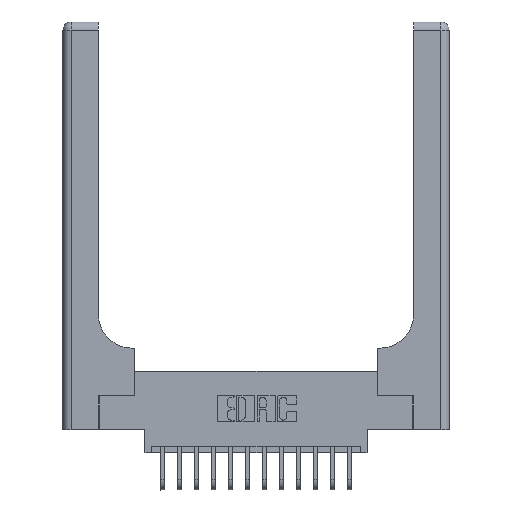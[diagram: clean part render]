
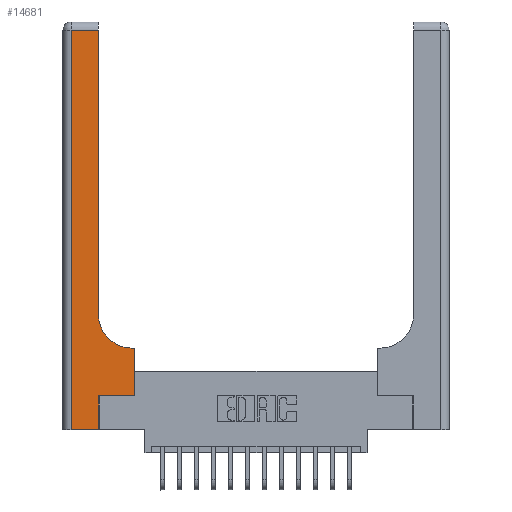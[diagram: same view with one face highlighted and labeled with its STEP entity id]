
A CAD part, top view. The second image highlights one B-rep face of the part: STEP entity #14681.
In plain terms, the highlighted planar face has unit normal (0, 0, 1).
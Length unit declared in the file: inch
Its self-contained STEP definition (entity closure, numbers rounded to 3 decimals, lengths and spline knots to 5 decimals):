
#209 = DIRECTION ( 'NONE',  ( -1., 0., 0. ) ) ;
#928 = CARTESIAN_POINT ( 'NONE',  ( 0., 2.94, 0.37 ) ) ;
#1192 = DIRECTION ( 'NONE',  ( 1., 0., 0. ) ) ;
#1313 = CARTESIAN_POINT ( 'NONE',  ( 0.26, 0.85, 0.37 ) ) ;
#1513 = CARTESIAN_POINT ( 'NONE',  ( 0.26, 3., 0.37 ) ) ;
#1604 = DIRECTION ( 'NONE',  ( 0., -1., 0. ) ) ;
#1934 = LINE ( 'NONE', #13010, #3086 ) ;
#2556 = VECTOR ( 'NONE', #18748, 39.37008 ) ;
#2613 = DIRECTION ( 'NONE',  ( 0., 1., 0. ) ) ;
#2670 = EDGE_CURVE ( 'NONE', #9535, #18361, #16892, .T. ) ;
#2828 = VECTOR ( 'NONE', #11881, 39.37008 ) ;
#3066 = PLANE ( 'NONE',  #6196 ) ;
#3086 = VECTOR ( 'NONE', #2613, 39.37008 ) ;
#3102 = VECTOR ( 'NONE', #6952, 39.37008 ) ;
#3120 = LINE ( 'NONE', #7701, #16442 ) ;
#3555 = ORIENTED_EDGE ( 'NONE', *, *, #8176, .T. ) ;
#3641 = VERTEX_POINT ( 'NONE', #9939 ) ;
#4040 = CARTESIAN_POINT ( 'NONE',  ( 0.528, 0.25, 0.37 ) ) ;
#4149 = CARTESIAN_POINT ( 'NONE',  ( 0.06, 2.94, 0.37 ) ) ;
#4226 = LINE ( 'NONE', #6604, #12489 ) ;
#4505 = ORIENTED_EDGE ( 'NONE', *, *, #17049, .T. ) ;
#4785 = VECTOR ( 'NONE', #12562, 39.37008 ) ;
#5015 = CARTESIAN_POINT ( 'NONE',  ( 0.51, 0.6, 0.37 ) ) ;
#5158 = DIRECTION ( 'NONE',  ( -1., 0., 0. ) ) ;
#5807 = VERTEX_POINT ( 'NONE', #13353 ) ;
#6076 = VERTEX_POINT ( 'NONE', #16192 ) ;
#6196 = AXIS2_PLACEMENT_3D ( 'NONE', #7346, #13395, #209 ) ;
#6457 = VECTOR ( 'NONE', #1192, 39.37008 ) ;
#6515 = ORIENTED_EDGE ( 'NONE', *, *, #12387, .T. ) ;
#6604 = CARTESIAN_POINT ( 'NONE',  ( 0.26, 0.6, 0.37 ) ) ;
#6660 = ORIENTED_EDGE ( 'NONE', *, *, #16191, .T. ) ;
#6952 = DIRECTION ( 'NONE',  ( -1., 0., 0. ) ) ;
#7073 = ORIENTED_EDGE ( 'NONE', *, *, #16228, .T. ) ;
#7172 = ORIENTED_EDGE ( 'NONE', *, *, #15254, .T. ) ;
#7177 = CARTESIAN_POINT ( 'NONE',  ( 0.51, 0.85, 0.37 ) ) ;
#7240 = LINE ( 'NONE', #1513, #2828 ) ;
#7346 = CARTESIAN_POINT ( 'NONE',  ( 0., 3., 0.37 ) ) ;
#7701 = CARTESIAN_POINT ( 'NONE',  ( 0.06, 3., 0.37 ) ) ;
#7970 = VERTEX_POINT ( 'NONE', #8916 ) ;
#8176 = EDGE_CURVE ( 'NONE', #3641, #9535, #4226, .T. ) ;
#8916 = CARTESIAN_POINT ( 'NONE',  ( 0.26, 2.94, 0.37 ) ) ;
#8963 = VERTEX_POINT ( 'NONE', #16200 ) ;
#9535 = VERTEX_POINT ( 'NONE', #5015 ) ;
#9939 = CARTESIAN_POINT ( 'NONE',  ( 0.528, 0.6, 0.37 ) ) ;
#11642 = EDGE_CURVE ( 'NONE', #8963, #5807, #16741, .T. ) ;
#11881 = DIRECTION ( 'NONE',  ( 0., 1., 0. ) ) ;
#12387 = EDGE_CURVE ( 'NONE', #18439, #6076, #16718, .T. ) ;
#12489 = VECTOR ( 'NONE', #5158, 39.37008 ) ;
#12562 = DIRECTION ( 'NONE',  ( 1., 0., 0. ) ) ;
#13010 = CARTESIAN_POINT ( 'NONE',  ( 0.265, 0., 0.37 ) ) ;
#13167 = CARTESIAN_POINT ( 'NONE',  ( 0.06, 0., 0.37 ) ) ;
#13353 = CARTESIAN_POINT ( 'NONE',  ( 0.528, 0.25, 0.37 ) ) ;
#13395 = DIRECTION ( 'NONE',  ( 0., 0., -1. ) ) ;
#13799 = ORIENTED_EDGE ( 'NONE', *, *, #2670, .T. ) ;
#14381 = FACE_OUTER_BOUND ( 'NONE', #17236, .T. ) ;
#14610 = DIRECTION ( 'NONE',  ( 0., 0., -1. ) ) ;
#14681 = ADVANCED_FACE ( 'NONE', ( #14381 ), #3066, .F. ) ;
#14791 = LINE ( 'NONE', #928, #3102 ) ;
#15254 = EDGE_CURVE ( 'NONE', #16194, #18439, #3120, .T. ) ;
#16191 = EDGE_CURVE ( 'NONE', #7970, #16194, #14791, .T. ) ;
#16192 = CARTESIAN_POINT ( 'NONE',  ( 0.265, 0., 0.37 ) ) ;
#16194 = VERTEX_POINT ( 'NONE', #4149 ) ;
#16200 = CARTESIAN_POINT ( 'NONE',  ( 0.265, 0.25, 0.37 ) ) ;
#16211 = AXIS2_PLACEMENT_3D ( 'NONE', #7177, #14610, #17579 ) ;
#16228 = EDGE_CURVE ( 'NONE', #6076, #8963, #1934, .T. ) ;
#16442 = VECTOR ( 'NONE', #1604, 39.37008 ) ;
#16718 = LINE ( 'NONE', #17037, #4785 ) ;
#16741 = LINE ( 'NONE', #18709, #6457 ) ;
#16892 = CIRCLE ( 'NONE', #16211, 0.25 ) ;
#17037 = CARTESIAN_POINT ( 'NONE',  ( 0., 0., 0.37 ) ) ;
#17049 = EDGE_CURVE ( 'NONE', #18361, #7970, #7240, .T. ) ;
#17236 = EDGE_LOOP ( 'NONE', ( #4505, #6660, #7172, #6515, #7073, #17917, #18873, #3555, #13799 ) ) ;
#17579 = DIRECTION ( 'NONE',  ( 1., 0., 0. ) ) ;
#17917 = ORIENTED_EDGE ( 'NONE', *, *, #11642, .T. ) ;
#17944 = EDGE_CURVE ( 'NONE', #5807, #3641, #18592, .T. ) ;
#18361 = VERTEX_POINT ( 'NONE', #1313 ) ;
#18439 = VERTEX_POINT ( 'NONE', #13167 ) ;
#18592 = LINE ( 'NONE', #4040, #2556 ) ;
#18709 = CARTESIAN_POINT ( 'NONE',  ( 0.265, 0.25, 0.37 ) ) ;
#18748 = DIRECTION ( 'NONE',  ( 0., 1., 0. ) ) ;
#18873 = ORIENTED_EDGE ( 'NONE', *, *, #17944, .T. ) ;
